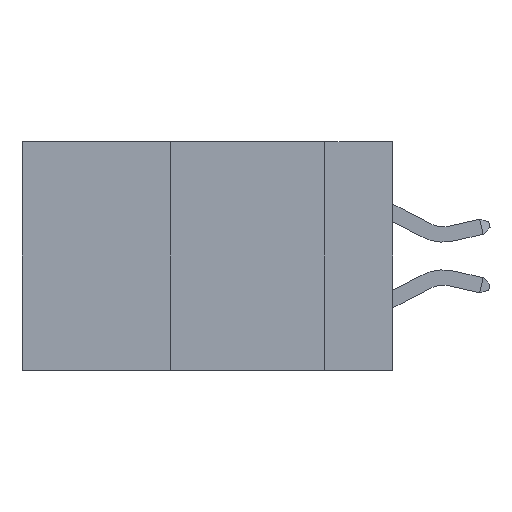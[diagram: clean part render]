
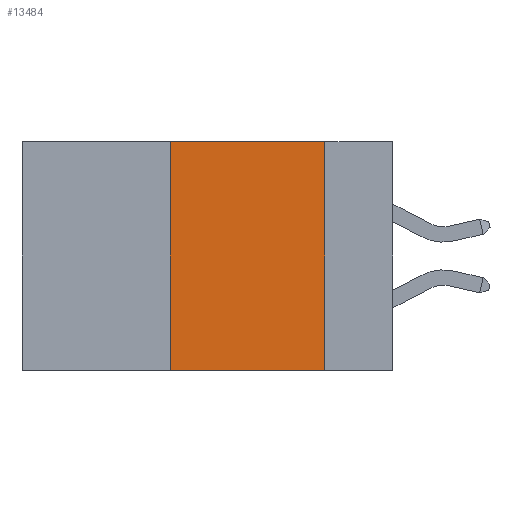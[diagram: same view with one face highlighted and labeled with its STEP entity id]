
A CAD part, left-side view. The second image highlights one B-rep face of the part: STEP entity #13484.
In plain terms, the highlighted planar face has unit normal (-1, 0, 0).
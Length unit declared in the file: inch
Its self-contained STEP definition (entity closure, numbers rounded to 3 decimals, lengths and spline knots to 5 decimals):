
#35 = CARTESIAN_POINT ( 'NONE',  ( 0., 0.6, 0. ) ) ;
#274 = VERTEX_POINT ( 'NONE', #11240 ) ;
#1202 = DIRECTION ( 'NONE',  ( 1., 0., 0. ) ) ;
#1355 = AXIS2_PLACEMENT_3D ( 'NONE', #35, #1202, #8748 ) ;
#1506 = DIRECTION ( 'NONE',  ( 0., 0., 1. ) ) ;
#1553 = EDGE_CURVE ( 'NONE', #5876, #14166, #6751, .T. ) ;
#1679 = VECTOR ( 'NONE', #11164, 39.37008 ) ;
#2762 = CARTESIAN_POINT ( 'NONE',  ( 0., 0.11, -0.37 ) ) ;
#3247 = ORIENTED_EDGE ( 'NONE', *, *, #4459, .F. ) ;
#3289 = PLANE ( 'NONE',  #1355 ) ;
#3594 = CARTESIAN_POINT ( 'NONE',  ( 0., 0.36, 0. ) ) ;
#3917 = CARTESIAN_POINT ( 'NONE',  ( 0., 0.6, 0. ) ) ;
#4063 = LINE ( 'NONE', #3917, #11465 ) ;
#4459 = EDGE_CURVE ( 'NONE', #274, #14166, #13514, .T. ) ;
#4627 = VECTOR ( 'NONE', #7003, 39.37008 ) ;
#4782 = CARTESIAN_POINT ( 'NONE',  ( 0., 0.36, 0. ) ) ;
#5876 = VERTEX_POINT ( 'NONE', #8526 ) ;
#6751 = LINE ( 'NONE', #12457, #1679 ) ;
#7003 = DIRECTION ( 'NONE',  ( 0., 0., -1. ) ) ;
#7158 = EDGE_CURVE ( 'NONE', #5876, #14040, #13605, .T. ) ;
#7343 = ORIENTED_EDGE ( 'NONE', *, *, #13761, .F. ) ;
#8448 = DIRECTION ( 'NONE',  ( 0., -1., 0. ) ) ;
#8526 = CARTESIAN_POINT ( 'NONE',  ( 0., 0.36, -0.37 ) ) ;
#8748 = DIRECTION ( 'NONE',  ( 0., 0., -1. ) ) ;
#9097 = ORIENTED_EDGE ( 'NONE', *, *, #7158, .F. ) ;
#9242 = CARTESIAN_POINT ( 'NONE',  ( 0., 0.11, 0. ) ) ;
#9740 = VECTOR ( 'NONE', #1506, 39.37008 ) ;
#10024 = EDGE_LOOP ( 'NONE', ( #3247, #7343, #9097, #10596 ) ) ;
#10596 = ORIENTED_EDGE ( 'NONE', *, *, #1553, .T. ) ;
#11164 = DIRECTION ( 'NONE',  ( 0., -1., 0. ) ) ;
#11240 = CARTESIAN_POINT ( 'NONE',  ( 0., 0.11, 0. ) ) ;
#11465 = VECTOR ( 'NONE', #8448, 39.37008 ) ;
#12457 = CARTESIAN_POINT ( 'NONE',  ( 0., 0.6, -0.37 ) ) ;
#13007 = FACE_OUTER_BOUND ( 'NONE', #10024, .T. ) ;
#13484 = ADVANCED_FACE ( 'NONE', ( #13007 ), #3289, .F. ) ;
#13514 = LINE ( 'NONE', #9242, #4627 ) ;
#13605 = LINE ( 'NONE', #3594, #9740 ) ;
#13761 = EDGE_CURVE ( 'NONE', #14040, #274, #4063, .T. ) ;
#14040 = VERTEX_POINT ( 'NONE', #4782 ) ;
#14166 = VERTEX_POINT ( 'NONE', #2762 ) ;
